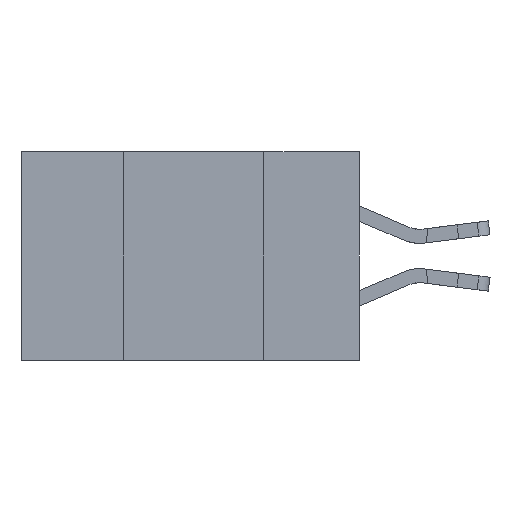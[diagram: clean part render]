
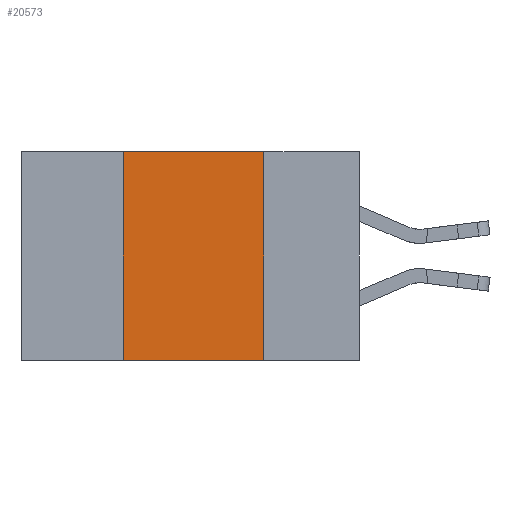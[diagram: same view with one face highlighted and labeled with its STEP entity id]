
A CAD part, left-side view. The second image highlights one B-rep face of the part: STEP entity #20573.
In plain terms, the highlighted planar face has unit normal (-1, 0, 0).
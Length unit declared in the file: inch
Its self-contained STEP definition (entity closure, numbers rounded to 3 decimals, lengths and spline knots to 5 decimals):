
#4 = VECTOR ( 'NONE', #11602, 39.37008 ) ;
#395 = LINE ( 'NONE', #9840, #10056 ) ;
#799 = PLANE ( 'NONE',  #25236 ) ;
#2633 = ORIENTED_EDGE ( 'NONE', *, *, #30988, .F. ) ;
#2924 = ORIENTED_EDGE ( 'NONE', *, *, #29515, .T. ) ;
#3577 = CARTESIAN_POINT ( 'NONE',  ( 0., 0.17, 0. ) ) ;
#3600 = DIRECTION ( 'NONE',  ( 0., 0., -1. ) ) ;
#4268 = CARTESIAN_POINT ( 'NONE',  ( 0., 0.42, 0. ) ) ;
#4494 = VECTOR ( 'NONE', #20041, 39.37008 ) ;
#5979 = VERTEX_POINT ( 'NONE', #4268 ) ;
#6448 = LINE ( 'NONE', #19812, #4494 ) ;
#7141 = VERTEX_POINT ( 'NONE', #3577 ) ;
#8309 = LINE ( 'NONE', #31270, #4 ) ;
#8536 = FACE_OUTER_BOUND ( 'NONE', #11261, .T. ) ;
#8729 = EDGE_CURVE ( 'NONE', #5979, #7141, #27889, .T. ) ;
#9840 = CARTESIAN_POINT ( 'NONE',  ( 0., 0.17, 0. ) ) ;
#10056 = VECTOR ( 'NONE', #29612, 39.37008 ) ;
#10821 = CARTESIAN_POINT ( 'NONE',  ( 0., 0.42, -0.37 ) ) ;
#11156 = CARTESIAN_POINT ( 'NONE',  ( 0., 0.6, 0. ) ) ;
#11261 = EDGE_LOOP ( 'NONE', ( #2633, #13264, #22549, #2924 ) ) ;
#11602 = DIRECTION ( 'NONE',  ( 0., 0., 1. ) ) ;
#13264 = ORIENTED_EDGE ( 'NONE', *, *, #8729, .F. ) ;
#14878 = VECTOR ( 'NONE', #22471, 39.37008 ) ;
#18048 = CARTESIAN_POINT ( 'NONE',  ( 0., 0.6, 0. ) ) ;
#18244 = VERTEX_POINT ( 'NONE', #21275 ) ;
#19812 = CARTESIAN_POINT ( 'NONE',  ( 0., 0.6, -0.37 ) ) ;
#20041 = DIRECTION ( 'NONE',  ( 0., -1., 0. ) ) ;
#20573 = ADVANCED_FACE ( 'NONE', ( #8536 ), #799, .F. ) ;
#21275 = CARTESIAN_POINT ( 'NONE',  ( 0., 0.17, -0.37 ) ) ;
#22471 = DIRECTION ( 'NONE',  ( 0., -1., 0. ) ) ;
#22549 = ORIENTED_EDGE ( 'NONE', *, *, #32251, .F. ) ;
#25236 = AXIS2_PLACEMENT_3D ( 'NONE', #11156, #28636, #3600 ) ;
#27889 = LINE ( 'NONE', #18048, #14878 ) ;
#28636 = DIRECTION ( 'NONE',  ( 1., 0., 0. ) ) ;
#29515 = EDGE_CURVE ( 'NONE', #32035, #18244, #6448, .T. ) ;
#29612 = DIRECTION ( 'NONE',  ( 0., 0., -1. ) ) ;
#30988 = EDGE_CURVE ( 'NONE', #7141, #18244, #395, .T. ) ;
#31270 = CARTESIAN_POINT ( 'NONE',  ( 0., 0.42, 0. ) ) ;
#32035 = VERTEX_POINT ( 'NONE', #10821 ) ;
#32251 = EDGE_CURVE ( 'NONE', #32035, #5979, #8309, .T. ) ;
